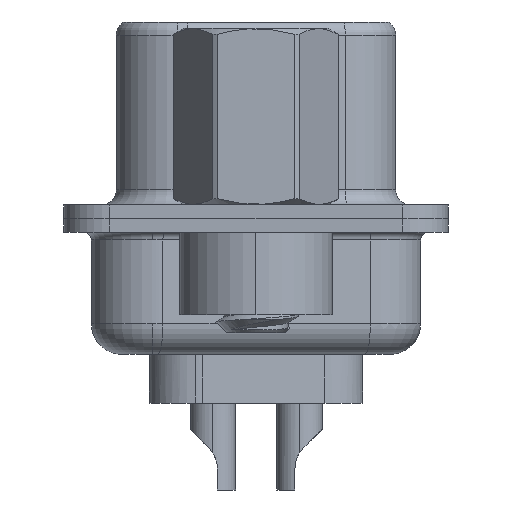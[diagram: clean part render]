
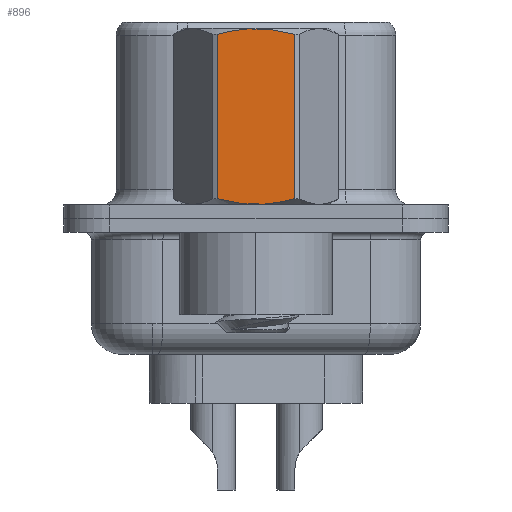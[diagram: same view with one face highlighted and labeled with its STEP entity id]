
A CAD part, left-side view. The second image highlights one B-rep face of the part: STEP entity #896.
In plain terms, the highlighted planar face has unit normal (-1, 0, 0).
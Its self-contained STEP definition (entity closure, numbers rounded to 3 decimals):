
#368 = VERTEX_POINT ( 'NONE', #6028 ) ;
#796 = CARTESIAN_POINT ( 'NONE',  ( -2.381, -1.273, 0.652 ) ) ;
#896 = ADVANCED_FACE ( 'NONE', ( #1089 ), #12656, .T. ) ;
#1089 = FACE_OUTER_BOUND ( 'NONE', #13632, .T. ) ;
#1440 = ORIENTED_EDGE ( 'NONE', *, *, #3831, .T. ) ;
#1442 = CARTESIAN_POINT ( 'NONE',  ( -2.381, 1.273, 3.792 ) ) ;
#1472 = CARTESIAN_POINT ( 'NONE',  ( -2.381, -0.858, 6.15 ) ) ;
#1818 = VERTEX_POINT ( 'NONE', #14526 ) ;
#3109 = DIRECTION ( 'NONE',  ( 0., 0., -1. ) ) ;
#3153 = B_SPLINE_CURVE_WITH_KNOTS ( 'NONE', 3,
 ( #8029, #19458, #1472, #8274, #8106, #14933, #8247, #8178, #20781, #20776 ),
 .UNSPECIFIED., .F., .F.,
 ( 4, 2, 2, 2, 4 ),
 ( 0.001, 0.002, 0.002, 0.003, 0.004 ),
 .UNSPECIFIED. ) ;
#3274 = CARTESIAN_POINT ( 'NONE',  ( -2.381, -0.432, 0.485 ) ) ;
#3484 = VECTOR ( 'NONE', #14109, 1000. ) ;
#3549 = EDGE_CURVE ( 'NONE', #368, #16287, #3153, .T. ) ;
#3831 = EDGE_CURVE ( 'NONE', #1818, #17163, #9536, .T. ) ;
#4228 = CARTESIAN_POINT ( 'NONE',  ( -2.381, 1.273, 6.048 ) ) ;
#4907 = AXIS2_PLACEMENT_3D ( 'NONE', #13886, #19289, #18758 ) ;
#4942 = LINE ( 'NONE', #1442, #8720 ) ;
#6028 = CARTESIAN_POINT ( 'NONE',  ( -2.381, -1.273, 6.048 ) ) ;
#6044 = CARTESIAN_POINT ( 'NONE',  ( -2.381, -1.273, 3.792 ) ) ;
#8029 = CARTESIAN_POINT ( 'NONE',  ( -2.381, -1.273, 6.048 ) ) ;
#8106 = CARTESIAN_POINT ( 'NONE',  ( -2.381, -0.215, 6.232 ) ) ;
#8178 = CARTESIAN_POINT ( 'NONE',  ( -2.381, 0.853, 6.151 ) ) ;
#8247 = CARTESIAN_POINT ( 'NONE',  ( -2.381, 0.428, 6.215 ) ) ;
#8274 = CARTESIAN_POINT ( 'NONE',  ( -2.381, -0.432, 6.215 ) ) ;
#8720 = VECTOR ( 'NONE', #3109, 1000. ) ;
#9536 = B_SPLINE_CURVE_WITH_KNOTS ( 'NONE', 3,
 ( #10760, #10809, #20943, #11220, #20087, #11624, #3274, #19270, #19082, #19057 ),
 .UNSPECIFIED., .F., .F.,
 ( 4, 2, 2, 2, 4 ),
 ( 0.003, 0.003, 0.004, 0.004, 0.005 ),
 .UNSPECIFIED. ) ;
#10031 = EDGE_CURVE ( 'NONE', #16287, #1818, #4942, .T. ) ;
#10760 = CARTESIAN_POINT ( 'NONE',  ( -2.381, 1.273, 0.652 ) ) ;
#10809 = CARTESIAN_POINT ( 'NONE',  ( -2.381, 1.065, 0.596 ) ) ;
#11220 = CARTESIAN_POINT ( 'NONE',  ( -2.381, 0.428, 0.485 ) ) ;
#11624 = CARTESIAN_POINT ( 'NONE',  ( -2.381, -0.215, 0.468 ) ) ;
#11787 = ORIENTED_EDGE ( 'NONE', *, *, #10031, .T. ) ;
#12656 = PLANE ( 'NONE',  #4907 ) ;
#13248 = EDGE_CURVE ( 'NONE', #17163, #368, #13569, .T. ) ;
#13569 = LINE ( 'NONE', #6044, #3484 ) ;
#13632 = EDGE_LOOP ( 'NONE', ( #1440, #20269, #18995, #11787 ) ) ;
#13886 = CARTESIAN_POINT ( 'NONE',  ( -2.381, 1.375, -3.75 ) ) ;
#14109 = DIRECTION ( 'NONE',  ( 0., 0., 1. ) ) ;
#14526 = CARTESIAN_POINT ( 'NONE',  ( -2.381, 1.273, 0.652 ) ) ;
#14933 = CARTESIAN_POINT ( 'NONE',  ( -2.381, 0.215, 6.232 ) ) ;
#16287 = VERTEX_POINT ( 'NONE', #4228 ) ;
#17163 = VERTEX_POINT ( 'NONE', #796 ) ;
#18758 = DIRECTION ( 'NONE',  ( 0., -1., 0. ) ) ;
#18995 = ORIENTED_EDGE ( 'NONE', *, *, #3549, .T. ) ;
#19057 = CARTESIAN_POINT ( 'NONE',  ( -2.381, -1.273, 0.652 ) ) ;
#19082 = CARTESIAN_POINT ( 'NONE',  ( -2.381, -1.066, 0.596 ) ) ;
#19270 = CARTESIAN_POINT ( 'NONE',  ( -2.381, -0.858, 0.55 ) ) ;
#19289 = DIRECTION ( 'NONE',  ( -1., 0., 0. ) ) ;
#19458 = CARTESIAN_POINT ( 'NONE',  ( -2.381, -1.066, 6.104 ) ) ;
#20087 = CARTESIAN_POINT ( 'NONE',  ( -2.381, 0.215, 0.468 ) ) ;
#20269 = ORIENTED_EDGE ( 'NONE', *, *, #13248, .T. ) ;
#20776 = CARTESIAN_POINT ( 'NONE',  ( -2.381, 1.273, 6.048 ) ) ;
#20781 = CARTESIAN_POINT ( 'NONE',  ( -2.381, 1.065, 6.104 ) ) ;
#20943 = CARTESIAN_POINT ( 'NONE',  ( -2.381, 0.853, 0.549 ) ) ;
